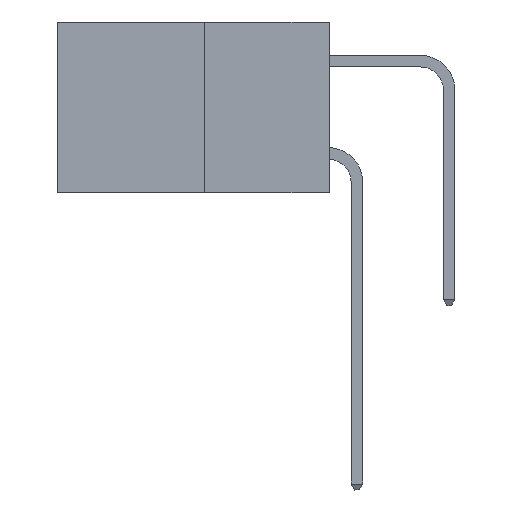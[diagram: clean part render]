
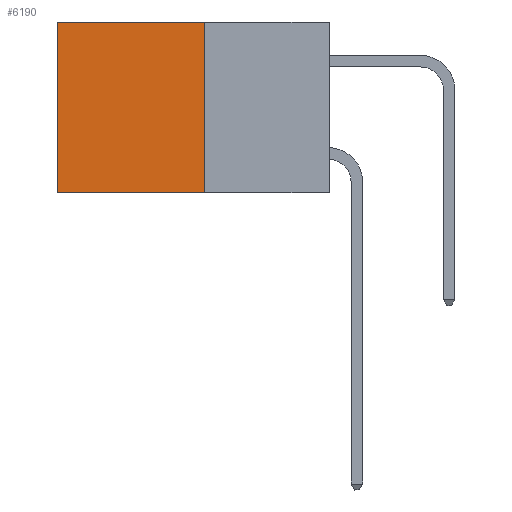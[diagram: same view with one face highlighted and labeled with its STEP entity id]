
A CAD part, left-side view. The second image highlights one B-rep face of the part: STEP entity #6190.
In plain terms, the highlighted planar face has unit normal (-1, 0, 0).
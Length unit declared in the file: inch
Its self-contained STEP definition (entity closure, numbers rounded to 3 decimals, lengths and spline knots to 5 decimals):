
#21 = CARTESIAN_POINT ( 'NONE',  ( 0.277, 0.27, -0.37 ) ) ;
#48 = CARTESIAN_POINT ( 'NONE',  ( 0.277, 0.27, 0. ) ) ;
#79 = DIRECTION ( 'NONE',  ( 0., 1., 0. ) ) ;
#157 = EDGE_CURVE ( 'NONE', #10385, #9283, #7943, .T. ) ;
#351 = LINE ( 'NONE', #48, #7794 ) ;
#556 = EDGE_CURVE ( 'NONE', #9305, #9283, #3166, .T. ) ;
#574 = EDGE_CURVE ( 'NONE', #9719, #10385, #351, .T. ) ;
#955 = CARTESIAN_POINT ( 'NONE',  ( 0.277, 0.59, -0.37 ) ) ;
#1811 = DIRECTION ( 'NONE',  ( 1., 0., 0. ) ) ;
#1837 = DIRECTION ( 'NONE',  ( 0., 1., 0. ) ) ;
#2446 = FACE_OUTER_BOUND ( 'NONE', #11261, .T. ) ;
#2705 = CARTESIAN_POINT ( 'NONE',  ( 0.277, 0.27, -0.37 ) ) ;
#3166 = LINE ( 'NONE', #21, #5310 ) ;
#3294 = VECTOR ( 'NONE', #11444, 39.37008 ) ;
#3479 = CARTESIAN_POINT ( 'NONE',  ( 0.277, 0.27, 0. ) ) ;
#4632 = CARTESIAN_POINT ( 'NONE',  ( 0.277, 0.27, -0.37 ) ) ;
#5310 = VECTOR ( 'NONE', #1837, 39.37008 ) ;
#5466 = PLANE ( 'NONE',  #11110 ) ;
#6047 = LINE ( 'NONE', #11410, #3294 ) ;
#6190 = ADVANCED_FACE ( 'NONE', ( #2446 ), #5466, .F. ) ;
#6564 = EDGE_CURVE ( 'NONE', #9719, #9305, #6047, .T. ) ;
#7352 = VECTOR ( 'NONE', #9432, 39.37008 ) ;
#7794 = VECTOR ( 'NONE', #79, 39.37008 ) ;
#7943 = LINE ( 'NONE', #9395, #7352 ) ;
#8256 = DIRECTION ( 'NONE',  ( 0., 0., -1. ) ) ;
#8381 = ORIENTED_EDGE ( 'NONE', *, *, #157, .T. ) ;
#8675 = ORIENTED_EDGE ( 'NONE', *, *, #6564, .F. ) ;
#9283 = VERTEX_POINT ( 'NONE', #955 ) ;
#9305 = VERTEX_POINT ( 'NONE', #4632 ) ;
#9395 = CARTESIAN_POINT ( 'NONE',  ( 0.277, 0.59, -0.37 ) ) ;
#9432 = DIRECTION ( 'NONE',  ( 0., 0., -1. ) ) ;
#9719 = VERTEX_POINT ( 'NONE', #3479 ) ;
#9986 = CARTESIAN_POINT ( 'NONE',  ( 0.277, 0.59, 0. ) ) ;
#10385 = VERTEX_POINT ( 'NONE', #9986 ) ;
#10776 = ORIENTED_EDGE ( 'NONE', *, *, #556, .F. ) ;
#11047 = ORIENTED_EDGE ( 'NONE', *, *, #574, .T. ) ;
#11110 = AXIS2_PLACEMENT_3D ( 'NONE', #2705, #1811, #8256 ) ;
#11261 = EDGE_LOOP ( 'NONE', ( #8381, #10776, #8675, #11047 ) ) ;
#11410 = CARTESIAN_POINT ( 'NONE',  ( 0.277, 0.27, -0.37 ) ) ;
#11444 = DIRECTION ( 'NONE',  ( 0., 0., -1. ) ) ;
